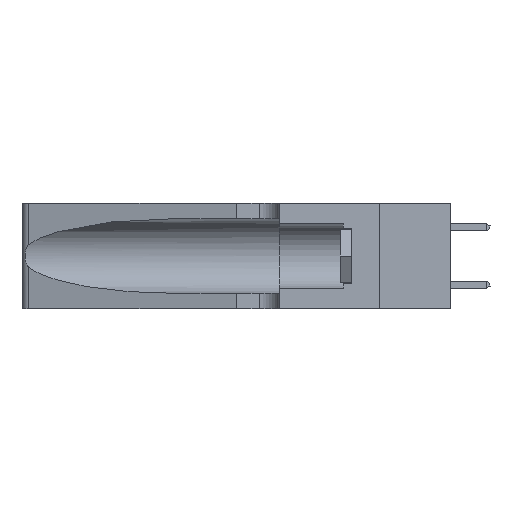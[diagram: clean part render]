
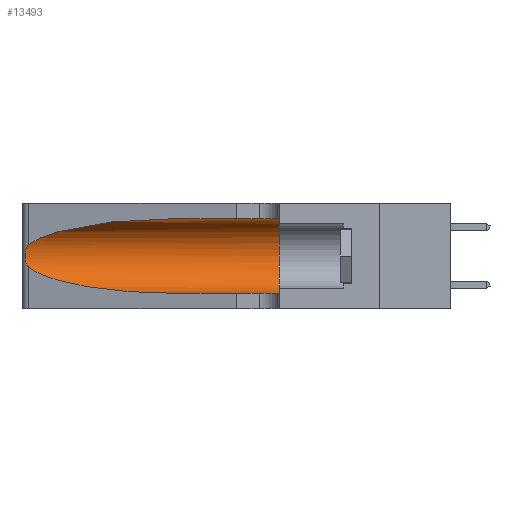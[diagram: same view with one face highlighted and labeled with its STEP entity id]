
A CAD part, left-side view. The second image highlights one B-rep face of the part: STEP entity #13493.
In plain terms, the highlighted cylindrical face has radius 3.308 mm (diameter 6.617 mm), a partial arc.
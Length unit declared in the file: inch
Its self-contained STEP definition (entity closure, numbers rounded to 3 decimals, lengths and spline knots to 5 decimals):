
#275 = CARTESIAN_POINT ( 'NONE',  ( 0.25487, 1.22718, 0.14631 ) ) ;
#581 = CARTESIAN_POINT ( 'NONE',  ( 0.1305, 1.61858, 0.185 ) ) ;
#641 = CARTESIAN_POINT ( 'NONE',  ( 0.26018, 1.23835, 0.19895 ) ) ;
#733 = VERTEX_POINT ( 'NONE', #10782 ) ;
#1089 = CYLINDRICAL_SURFACE ( 'NONE', #10636, 0.13025 ) ;
#1449 = ORIENTED_EDGE ( 'NONE', *, *, #9652, .F. ) ;
#1888 = CARTESIAN_POINT ( 'NONE',  ( 0.1305, 0.35, 0.185 ) ) ;
#1890 = CARTESIAN_POINT ( 'NONE',  ( 0.25487, 1.22718, 0.22369 ) ) ;
#1963 = CARTESIAN_POINT ( 'NONE',  ( 0.1305, 1.61858, 0.05475 ) ) ;
#2169 = EDGE_CURVE ( 'NONE', #733, #7028, #11873, .T. ) ;
#2775 = CARTESIAN_POINT ( 'NONE',  ( 0.18966, 0.96281, 0.05475 ) ) ;
#3446 = CARTESIAN_POINT ( 'NONE',  ( 0.1305, 0.35, 0.31525 ) ) ;
#3967 = AXIS2_PLACEMENT_3D ( 'NONE', #1888, #7423, #11046 ) ;
#4783 = VERTEX_POINT ( 'NONE', #8351 ) ;
#5557 = EDGE_CURVE ( 'NONE', #6935, #4783, #12928, .T. ) ;
#5624 = EDGE_CURVE ( 'NONE', #22100, #11351, #14359, .T. ) ;
#5642 = VECTOR ( 'NONE', #15278, 39.37008 ) ;
#5935 = CARTESIAN_POINT ( 'NONE',  ( 0.26075, 1.23896, 0.178 ) ) ;
#6005 = DIRECTION ( 'NONE',  ( 0., -1., 0. ) ) ;
#6495 = CARTESIAN_POINT ( 'NONE',  ( 0.1305, 0.72297, 0.05475 ) ) ;
#6935 = VERTEX_POINT ( 'NONE', #3446 ) ;
#7028 = VERTEX_POINT ( 'NONE', #20106 ) ;
#7423 = DIRECTION ( 'NONE',  ( 0., 1., 0. ) ) ;
#8002 = CARTESIAN_POINT ( 'NONE',  ( 0.25639, 1.23186, 0.15144 ) ) ;
#8231 = ORIENTED_EDGE ( 'NONE', *, *, #5624, .T. ) ;
#8351 = CARTESIAN_POINT ( 'NONE',  ( 0.1305, 0.35, 0.05475 ) ) ;
#8603 = ORIENTED_EDGE ( 'NONE', *, *, #10250, .T. ) ;
#9387 = CARTESIAN_POINT ( 'NONE',  ( 0.1305, 0.72297, 0.05475 ) ) ;
#9652 = EDGE_CURVE ( 'NONE', #733, #6935, #22317, .T. ) ;
#9802 = CARTESIAN_POINT ( 'NONE',  ( 0.25854, 1.2359, 0.20912 ) ) ;
#9886 = CARTESIAN_POINT ( 'NONE',  ( 0.25555, 1.22993, 0.14849 ) ) ;
#10034 = CARTESIAN_POINT ( 'NONE',  ( 0.2373, 1.15595, 0.08982 ) ) ;
#10250 = EDGE_CURVE ( 'NONE', #11351, #4783, #21476, .T. ) ;
#10636 = AXIS2_PLACEMENT_3D ( 'NONE', #581, #15142, #22358 ) ;
#10782 = CARTESIAN_POINT ( 'NONE',  ( 0.1305, 0.72297, 0.31525 ) ) ;
#11046 = DIRECTION ( 'NONE',  ( 0., 0., 1. ) ) ;
#11351 = VERTEX_POINT ( 'NONE', #9387 ) ;
#11380 = CARTESIAN_POINT ( 'NONE',  ( 0.25856, 1.23593, 0.16098 ) ) ;
#11465 = CARTESIAN_POINT ( 'NONE',  ( 0.25787, 1.23484, 0.2124 ) ) ;
#11705 = CARTESIAN_POINT ( 'NONE',  ( 0.25555, 1.22994, 0.2215 ) ) ;
#11873 =( BOUNDED_CURVE ( )  B_SPLINE_CURVE ( 3, ( #19716, #19897, #22097, #21594 ),
 .UNSPECIFIED., .F., .T. ) 
 B_SPLINE_CURVE_WITH_KNOTS ( ( 4, 4 ),
 ( 1.5708, 2.84003 ),
 .UNSPECIFIED. ) 
 CURVE ( )  GEOMETRIC_REPRESENTATION_ITEM ( )  RATIONAL_B_SPLINE_CURVE ( ( 1., 0.87, 0.87, 1. ) ) 
 REPRESENTATION_ITEM ( '' )  );
#12816 = CARTESIAN_POINT ( 'NONE',  ( 0.25639, 1.23184, 0.21858 ) ) ;
#12928 = CIRCLE ( 'NONE', #3967, 0.13025 ) ;
#13493 = ADVANCED_FACE ( 'NONE', ( #20734 ), #1089, .F. ) ;
#14359 =( BOUNDED_CURVE ( )  B_SPLINE_CURVE ( 3, ( #19015, #10034, #2775, #6495 ),
 .UNSPECIFIED., .F., .F. ) 
 B_SPLINE_CURVE_WITH_KNOTS ( ( 4, 4 ),
 ( 3.44316, 4.71239 ),
 .UNSPECIFIED. ) 
 CURVE ( )  GEOMETRIC_REPRESENTATION_ITEM ( )  RATIONAL_B_SPLINE_CURVE ( ( 1., 0.87, 0.87, 1. ) ) 
 REPRESENTATION_ITEM ( '' )  );
#14997 = ORIENTED_EDGE ( 'NONE', *, *, #20171, .T. ) ;
#15142 = DIRECTION ( 'NONE',  ( 0., -1., 0. ) ) ;
#15278 = DIRECTION ( 'NONE',  ( 0., -1., 0. ) ) ;
#15862 = ORIENTED_EDGE ( 'NONE', *, *, #2169, .T. ) ;
#16757 = CARTESIAN_POINT ( 'NONE',  ( 0.25487, 1.22718, 0.14631 ) ) ;
#16911 = CARTESIAN_POINT ( 'NONE',  ( 0.26075, 1.23896, 0.19203 ) ) ;
#16991 = CARTESIAN_POINT ( 'NONE',  ( 0.25789, 1.23486, 0.15765 ) ) ;
#17906 = CARTESIAN_POINT ( 'NONE',  ( 0.1305, 1.61858, 0.31525 ) ) ;
#18348 = VECTOR ( 'NONE', #6005, 39.37008 ) ;
#19015 = CARTESIAN_POINT ( 'NONE',  ( 0.25487, 1.22718, 0.14631 ) ) ;
#19716 = CARTESIAN_POINT ( 'NONE',  ( 0.1305, 0.72297, 0.31525 ) ) ;
#19897 = CARTESIAN_POINT ( 'NONE',  ( 0.18966, 0.96281, 0.31525 ) ) ;
#20106 = CARTESIAN_POINT ( 'NONE',  ( 0.25487, 1.22718, 0.22369 ) ) ;
#20171 = EDGE_CURVE ( 'NONE', #7028, #22100, #21252, .T. ) ;
#20477 = EDGE_LOOP ( 'NONE', ( #15862, #14997, #8231, #8603, #20586, #1449 ) ) ;
#20586 = ORIENTED_EDGE ( 'NONE', *, *, #5557, .F. ) ;
#20734 = FACE_OUTER_BOUND ( 'NONE', #20477, .T. ) ;
#21252 = B_SPLINE_CURVE_WITH_KNOTS ( 'NONE', 3,
 ( #1890, #11705, #12816, #11465, #9802, #641, #16911, #5935, #22185, #11380, #16991, #8002, #9886, #16757 ),
 .UNSPECIFIED., .F., .F.,
 ( 4, 2, 2, 2, 2, 2, 4 ),
 ( 0., 0.00027, 0.00053, 0.00107, 0.0016, 0.00187, 0.00214 ),
 .UNSPECIFIED. ) ;
#21476 = LINE ( 'NONE', #1963, #18348 ) ;
#21594 = CARTESIAN_POINT ( 'NONE',  ( 0.25487, 1.22718, 0.22369 ) ) ;
#22097 = CARTESIAN_POINT ( 'NONE',  ( 0.2373, 1.15595, 0.28018 ) ) ;
#22100 = VERTEX_POINT ( 'NONE', #275 ) ;
#22185 = CARTESIAN_POINT ( 'NONE',  ( 0.26017, 1.23833, 0.17102 ) ) ;
#22317 = LINE ( 'NONE', #17906, #5642 ) ;
#22358 = DIRECTION ( 'NONE',  ( 0., 0., -1. ) ) ;
